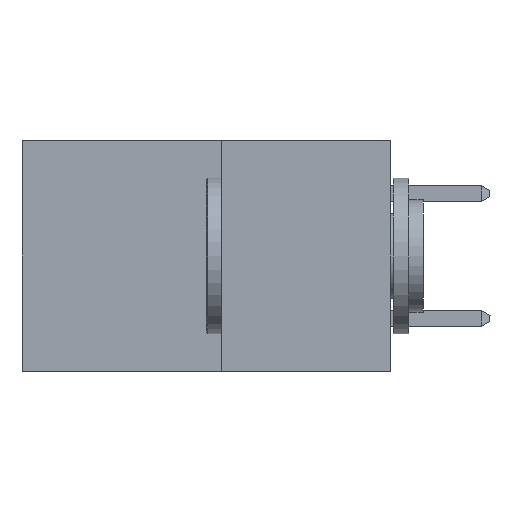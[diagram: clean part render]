
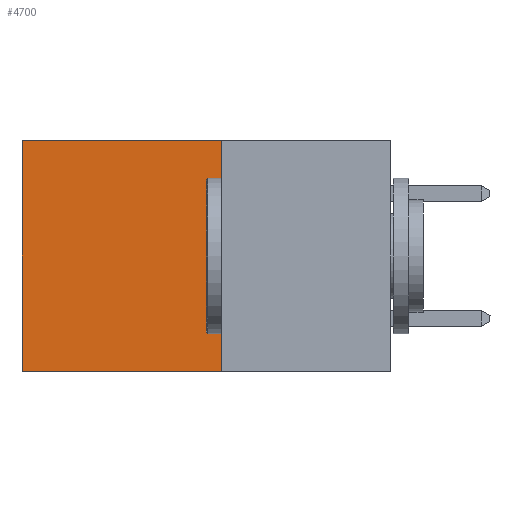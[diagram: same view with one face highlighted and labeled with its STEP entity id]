
A CAD part, left-side view. The second image highlights one B-rep face of the part: STEP entity #4700.
In plain terms, the highlighted planar face has unit normal (-1, 0, 0).
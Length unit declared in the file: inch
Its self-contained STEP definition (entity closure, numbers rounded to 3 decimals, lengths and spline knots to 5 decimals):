
#224 = CARTESIAN_POINT ( 'NONE',  ( 0.277, 0.27, -0.37 ) ) ;
#411 = EDGE_CURVE ( 'NONE', #6625, #6677, #9236, .T. ) ;
#550 = LINE ( 'NONE', #8099, #8950 ) ;
#744 = LINE ( 'NONE', #4825, #5109 ) ;
#1245 = CARTESIAN_POINT ( 'NONE',  ( 0.277, 0.59, 0. ) ) ;
#1336 = EDGE_LOOP ( 'NONE', ( #2737, #8957, #9189, #7496 ) ) ;
#1443 = EDGE_CURVE ( 'NONE', #4129, #2960, #744, .T. ) ;
#1835 = FACE_OUTER_BOUND ( 'NONE', #1336, .T. ) ;
#1894 = EDGE_CURVE ( 'NONE', #2960, #6677, #2186, .T. ) ;
#2121 = CARTESIAN_POINT ( 'NONE',  ( 0.277, 0.59, -0.37 ) ) ;
#2186 = LINE ( 'NONE', #2437, #8293 ) ;
#2437 = CARTESIAN_POINT ( 'NONE',  ( 0.277, 0.59, -0.37 ) ) ;
#2582 = DIRECTION ( 'NONE',  ( 0., 0., -1. ) ) ;
#2737 = ORIENTED_EDGE ( 'NONE', *, *, #1894, .T. ) ;
#2960 = VERTEX_POINT ( 'NONE', #1245 ) ;
#2961 = CARTESIAN_POINT ( 'NONE',  ( 0.277, 0.27, -0.37 ) ) ;
#3034 = VECTOR ( 'NONE', #7532, 39.37008 ) ;
#3187 = CARTESIAN_POINT ( 'NONE',  ( 0.277, 0.27, 0. ) ) ;
#3831 = PLANE ( 'NONE',  #3911 ) ;
#3911 = AXIS2_PLACEMENT_3D ( 'NONE', #224, #9211, #4670 ) ;
#4011 = DIRECTION ( 'NONE',  ( 0., 1., 0. ) ) ;
#4129 = VERTEX_POINT ( 'NONE', #3187 ) ;
#4360 = CARTESIAN_POINT ( 'NONE',  ( 0.277, 0.27, -0.37 ) ) ;
#4670 = DIRECTION ( 'NONE',  ( 0., 0., -1. ) ) ;
#4700 = ADVANCED_FACE ( 'NONE', ( #1835 ), #3831, .F. ) ;
#4825 = CARTESIAN_POINT ( 'NONE',  ( 0.277, 0.27, 0. ) ) ;
#5109 = VECTOR ( 'NONE', #4011, 39.37008 ) ;
#6625 = VERTEX_POINT ( 'NONE', #2961 ) ;
#6677 = VERTEX_POINT ( 'NONE', #2121 ) ;
#6905 = DIRECTION ( 'NONE',  ( 0., 0., -1. ) ) ;
#7205 = EDGE_CURVE ( 'NONE', #4129, #6625, #550, .T. ) ;
#7496 = ORIENTED_EDGE ( 'NONE', *, *, #1443, .T. ) ;
#7532 = DIRECTION ( 'NONE',  ( 0., 1., 0. ) ) ;
#8099 = CARTESIAN_POINT ( 'NONE',  ( 0.277, 0.27, -0.37 ) ) ;
#8293 = VECTOR ( 'NONE', #6905, 39.37008 ) ;
#8950 = VECTOR ( 'NONE', #2582, 39.37008 ) ;
#8957 = ORIENTED_EDGE ( 'NONE', *, *, #411, .F. ) ;
#9189 = ORIENTED_EDGE ( 'NONE', *, *, #7205, .F. ) ;
#9211 = DIRECTION ( 'NONE',  ( 1., 0., 0. ) ) ;
#9236 = LINE ( 'NONE', #4360, #3034 ) ;
